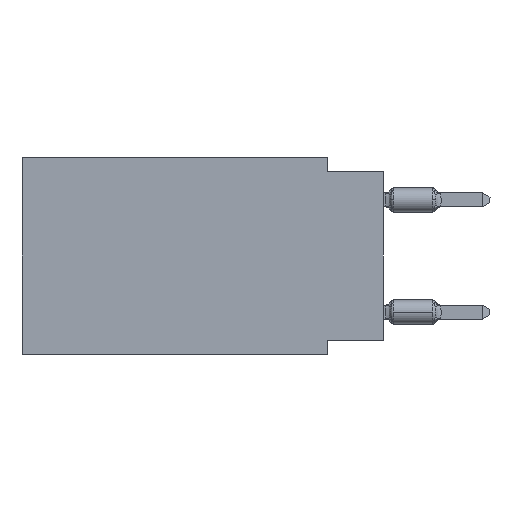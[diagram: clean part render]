
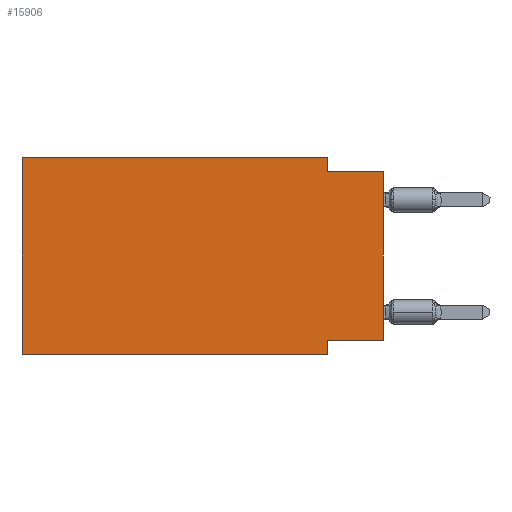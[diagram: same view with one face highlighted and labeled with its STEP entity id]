
A CAD part, left-side view. The second image highlights one B-rep face of the part: STEP entity #15906.
In plain terms, the highlighted planar face has unit normal (-1, 0, 0).
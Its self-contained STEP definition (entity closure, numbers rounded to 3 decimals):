
#311 = LINE ( 'NONE', #20735, #19553 ) ;
#416 = LINE ( 'NONE', #19000, #10343 ) ;
#629 = VECTOR ( 'NONE', #20704, 1000. ) ;
#723 = EDGE_CURVE ( 'NONE', #21938, #6714, #10416, .T. ) ;
#917 = CARTESIAN_POINT ( 'NONE',  ( 0., 2.54, -0.635 ) ) ;
#1123 = VECTOR ( 'NONE', #10810, 1000. ) ;
#1334 = VECTOR ( 'NONE', #7110, 1000. ) ;
#1403 = VERTEX_POINT ( 'NONE', #8295 ) ;
#1415 = EDGE_CURVE ( 'NONE', #7334, #10959, #13256, .T. ) ;
#1426 = ORIENTED_EDGE ( 'NONE', *, *, #1415, .F. ) ;
#1470 = EDGE_CURVE ( 'NONE', #21938, #17827, #20645, .T. ) ;
#1960 = EDGE_CURVE ( 'NONE', #1403, #12464, #416, .T. ) ;
#2026 = EDGE_CURVE ( 'NONE', #6714, #2669, #311, .T. ) ;
#2060 = CARTESIAN_POINT ( 'NONE',  ( 0., 16.383, 0. ) ) ;
#2669 = VERTEX_POINT ( 'NONE', #19246 ) ;
#2707 = EDGE_CURVE ( 'NONE', #12464, #17827, #16149, .T. ) ;
#3069 = EDGE_LOOP ( 'NONE', ( #18138, #10896, #18318, #6853, #1426, #22121, #19526, #18521 ) ) ;
#4590 = CARTESIAN_POINT ( 'NONE',  ( 0., 2.54, -8.255 ) ) ;
#5394 = DIRECTION ( 'NONE',  ( 1., 0., 0. ) ) ;
#6714 = VERTEX_POINT ( 'NONE', #4590 ) ;
#6853 = ORIENTED_EDGE ( 'NONE', *, *, #14138, .F. ) ;
#7110 = DIRECTION ( 'NONE',  ( 0., -1., 0. ) ) ;
#7189 = CARTESIAN_POINT ( 'NONE',  ( 0., 0., -8.255 ) ) ;
#7334 = VERTEX_POINT ( 'NONE', #16631 ) ;
#8061 = CARTESIAN_POINT ( 'NONE',  ( 0., 16.383, 0. ) ) ;
#8181 = DIRECTION ( 'NONE',  ( 0., 0., 1. ) ) ;
#8295 = CARTESIAN_POINT ( 'NONE',  ( 0., 2.54, 0. ) ) ;
#8823 = LINE ( 'NONE', #15884, #1334 ) ;
#9030 = DIRECTION ( 'NONE',  ( 0., 0., -1. ) ) ;
#10343 = VECTOR ( 'NONE', #9030, 1000. ) ;
#10416 = LINE ( 'NONE', #7189, #14770 ) ;
#10810 = DIRECTION ( 'NONE',  ( 0., -1., 0. ) ) ;
#10896 = ORIENTED_EDGE ( 'NONE', *, *, #2707, .F. ) ;
#10959 = VERTEX_POINT ( 'NONE', #15212 ) ;
#12464 = VERTEX_POINT ( 'NONE', #917 ) ;
#12531 = PLANE ( 'NONE',  #20515 ) ;
#13256 = LINE ( 'NONE', #8061, #17755 ) ;
#13646 = CARTESIAN_POINT ( 'NONE',  ( 0., 0., -0.635 ) ) ;
#14138 = EDGE_CURVE ( 'NONE', #10959, #1403, #15172, .T. ) ;
#14350 = DIRECTION ( 'NONE',  ( 0., 0., -1. ) ) ;
#14770 = VECTOR ( 'NONE', #17470, 1000. ) ;
#15172 = LINE ( 'NONE', #19087, #629 ) ;
#15212 = CARTESIAN_POINT ( 'NONE',  ( 0., 16.383, 0. ) ) ;
#15884 = CARTESIAN_POINT ( 'NONE',  ( 0., 16.383, -8.89 ) ) ;
#15906 = ADVANCED_FACE ( 'NONE', ( #18071 ), #12531, .F. ) ;
#16149 = LINE ( 'NONE', #21320, #1123 ) ;
#16631 = CARTESIAN_POINT ( 'NONE',  ( 0., 16.383, -8.89 ) ) ;
#17470 = DIRECTION ( 'NONE',  ( 0., 1., 0. ) ) ;
#17661 = CARTESIAN_POINT ( 'NONE',  ( 0., 0., -8.255 ) ) ;
#17755 = VECTOR ( 'NONE', #20534, 1000. ) ;
#17827 = VERTEX_POINT ( 'NONE', #13646 ) ;
#18071 = FACE_OUTER_BOUND ( 'NONE', #3069, .T. ) ;
#18138 = ORIENTED_EDGE ( 'NONE', *, *, #1470, .T. ) ;
#18318 = ORIENTED_EDGE ( 'NONE', *, *, #1960, .F. ) ;
#18521 = ORIENTED_EDGE ( 'NONE', *, *, #723, .F. ) ;
#18691 = CARTESIAN_POINT ( 'NONE',  ( 0., 0., 0. ) ) ;
#19000 = CARTESIAN_POINT ( 'NONE',  ( 0., 2.54, 0. ) ) ;
#19087 = CARTESIAN_POINT ( 'NONE',  ( 0., 16.383, 0. ) ) ;
#19246 = CARTESIAN_POINT ( 'NONE',  ( 0., 2.54, -8.89 ) ) ;
#19526 = ORIENTED_EDGE ( 'NONE', *, *, #2026, .F. ) ;
#19553 = VECTOR ( 'NONE', #14350, 1000. ) ;
#20515 = AXIS2_PLACEMENT_3D ( 'NONE', #2060, #5394, #21411 ) ;
#20534 = DIRECTION ( 'NONE',  ( 0., 0., 1. ) ) ;
#20645 = LINE ( 'NONE', #18691, #22526 ) ;
#20704 = DIRECTION ( 'NONE',  ( 0., -1., 0. ) ) ;
#20735 = CARTESIAN_POINT ( 'NONE',  ( 0., 2.54, -8.89 ) ) ;
#21176 = EDGE_CURVE ( 'NONE', #7334, #2669, #8823, .T. ) ;
#21320 = CARTESIAN_POINT ( 'NONE',  ( 0., 0., -0.635 ) ) ;
#21411 = DIRECTION ( 'NONE',  ( 0., 0., -1. ) ) ;
#21938 = VERTEX_POINT ( 'NONE', #17661 ) ;
#22121 = ORIENTED_EDGE ( 'NONE', *, *, #21176, .T. ) ;
#22526 = VECTOR ( 'NONE', #8181, 1000. ) ;
